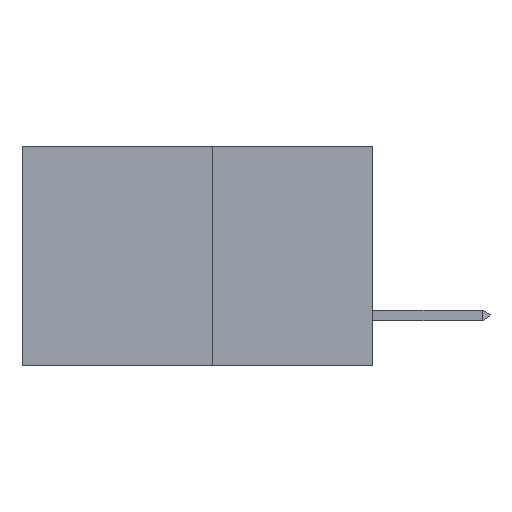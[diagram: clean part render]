
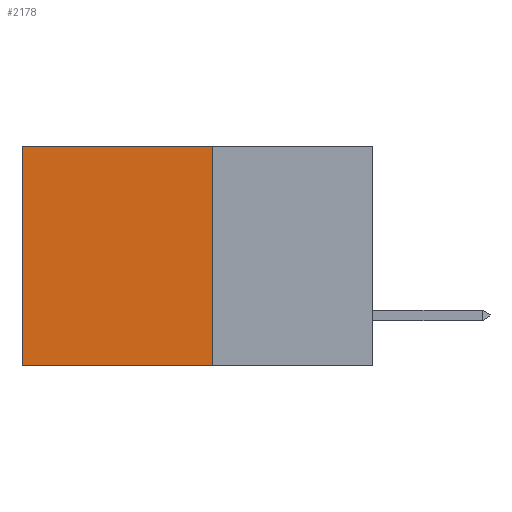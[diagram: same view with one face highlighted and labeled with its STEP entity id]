
A CAD part, left-side view. The second image highlights one B-rep face of the part: STEP entity #2178.
In plain terms, the highlighted planar face has unit normal (-1, 0, 0).
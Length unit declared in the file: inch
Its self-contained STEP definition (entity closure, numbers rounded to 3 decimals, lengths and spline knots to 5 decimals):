
#258 = EDGE_CURVE ( 'NONE', #2258, #5254, #5294, .T. ) ;
#1029 = DIRECTION ( 'NONE',  ( 0., 0., -1. ) ) ;
#1287 = ORIENTED_EDGE ( 'NONE', *, *, #4774, .T. ) ;
#1301 = ORIENTED_EDGE ( 'NONE', *, *, #9609, .F. ) ;
#1425 = CARTESIAN_POINT ( 'NONE',  ( 0.277, 0.59, -0.37 ) ) ;
#1638 = VERTEX_POINT ( 'NONE', #2650 ) ;
#1712 = PLANE ( 'NONE',  #3759 ) ;
#2178 = ADVANCED_FACE ( 'NONE', ( #4719 ), #1712, .F. ) ;
#2258 = VERTEX_POINT ( 'NONE', #4944 ) ;
#2650 = CARTESIAN_POINT ( 'NONE',  ( 0.277, 0.27, 0. ) ) ;
#2651 = VERTEX_POINT ( 'NONE', #8068 ) ;
#2731 = VECTOR ( 'NONE', #4407, 39.37008 ) ;
#2824 = ORIENTED_EDGE ( 'NONE', *, *, #5986, .T. ) ;
#3759 = AXIS2_PLACEMENT_3D ( 'NONE', #4002, #3940, #9055 ) ;
#3913 = LINE ( 'NONE', #7892, #7514 ) ;
#3940 = DIRECTION ( 'NONE',  ( 1., 0., 0. ) ) ;
#4002 = CARTESIAN_POINT ( 'NONE',  ( 0.277, 0.27, -0.37 ) ) ;
#4336 = ORIENTED_EDGE ( 'NONE', *, *, #258, .F. ) ;
#4407 = DIRECTION ( 'NONE',  ( 0., 0., -1. ) ) ;
#4454 = CARTESIAN_POINT ( 'NONE',  ( 0.277, 0.59, -0.37 ) ) ;
#4719 = FACE_OUTER_BOUND ( 'NONE', #5695, .T. ) ;
#4761 = LINE ( 'NONE', #4454, #2731 ) ;
#4774 = EDGE_CURVE ( 'NONE', #1638, #2651, #6122, .T. ) ;
#4944 = CARTESIAN_POINT ( 'NONE',  ( 0.277, 0.27, -0.37 ) ) ;
#5254 = VERTEX_POINT ( 'NONE', #1425 ) ;
#5294 = LINE ( 'NONE', #6764, #8819 ) ;
#5695 = EDGE_LOOP ( 'NONE', ( #2824, #4336, #1301, #1287 ) ) ;
#5986 = EDGE_CURVE ( 'NONE', #2651, #5254, #4761, .T. ) ;
#6122 = LINE ( 'NONE', #7741, #9610 ) ;
#6244 = DIRECTION ( 'NONE',  ( 0., 1., 0. ) ) ;
#6764 = CARTESIAN_POINT ( 'NONE',  ( 0.277, 0.27, -0.37 ) ) ;
#7514 = VECTOR ( 'NONE', #1029, 39.37008 ) ;
#7741 = CARTESIAN_POINT ( 'NONE',  ( 0.277, 0.27, 0. ) ) ;
#7762 = DIRECTION ( 'NONE',  ( 0., 1., 0. ) ) ;
#7892 = CARTESIAN_POINT ( 'NONE',  ( 0.277, 0.27, -0.37 ) ) ;
#8068 = CARTESIAN_POINT ( 'NONE',  ( 0.277, 0.59, 0. ) ) ;
#8819 = VECTOR ( 'NONE', #6244, 39.37008 ) ;
#9055 = DIRECTION ( 'NONE',  ( 0., 0., -1. ) ) ;
#9609 = EDGE_CURVE ( 'NONE', #1638, #2258, #3913, .T. ) ;
#9610 = VECTOR ( 'NONE', #7762, 39.37008 ) ;
